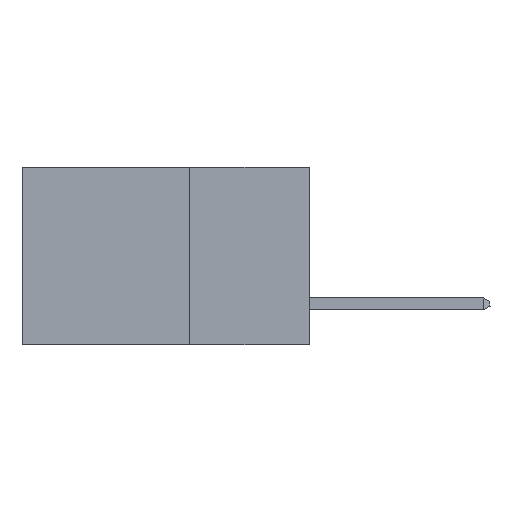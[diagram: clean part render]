
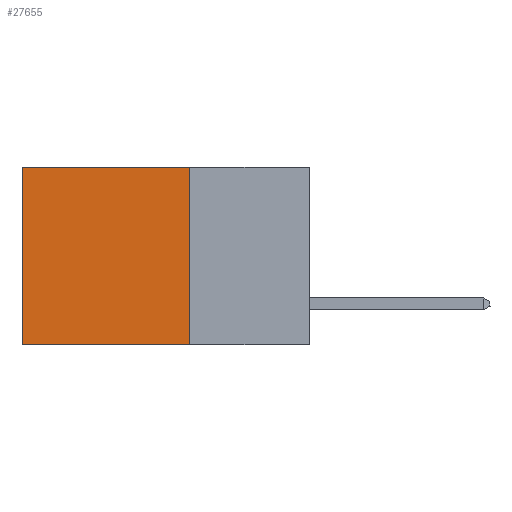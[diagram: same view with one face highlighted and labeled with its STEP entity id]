
A CAD part, left-side view. The second image highlights one B-rep face of the part: STEP entity #27655.
In plain terms, the highlighted planar face has unit normal (-1, 0, 0).
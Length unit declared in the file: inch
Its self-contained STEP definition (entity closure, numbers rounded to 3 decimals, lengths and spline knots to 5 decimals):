
#61 = LINE ( 'NONE', #29874, #7785 ) ;
#936 = EDGE_LOOP ( 'NONE', ( #32970, #7520, #23404, #4090 ) ) ;
#2208 = LINE ( 'NONE', #8037, #7498 ) ;
#3009 = VERTEX_POINT ( 'NONE', #13847 ) ;
#3869 = CARTESIAN_POINT ( 'NONE',  ( 0.2875, 0.25, -0.37 ) ) ;
#4090 = ORIENTED_EDGE ( 'NONE', *, *, #27673, .T. ) ;
#5864 = VECTOR ( 'NONE', #33023, 39.37008 ) ;
#5887 = AXIS2_PLACEMENT_3D ( 'NONE', #32640, #29722, #17159 ) ;
#6466 = VERTEX_POINT ( 'NONE', #9329 ) ;
#6578 = DIRECTION ( 'NONE',  ( 0., 1., 0. ) ) ;
#7107 = LINE ( 'NONE', #14974, #5864 ) ;
#7498 = VECTOR ( 'NONE', #31624, 39.37008 ) ;
#7520 = ORIENTED_EDGE ( 'NONE', *, *, #9804, .F. ) ;
#7785 = VECTOR ( 'NONE', #6578, 39.37008 ) ;
#8037 = CARTESIAN_POINT ( 'NONE',  ( 0.2875, 0.25, 0. ) ) ;
#8250 = LINE ( 'NONE', #16932, #19632 ) ;
#9329 = CARTESIAN_POINT ( 'NONE',  ( 0.2875, 0.6, 0. ) ) ;
#9804 = EDGE_CURVE ( 'NONE', #16215, #27872, #61, .T. ) ;
#13847 = CARTESIAN_POINT ( 'NONE',  ( 0.2875, 0.25, 0. ) ) ;
#14583 = PLANE ( 'NONE',  #5887 ) ;
#14974 = CARTESIAN_POINT ( 'NONE',  ( 0.2875, 0.6, 0. ) ) ;
#15435 = CARTESIAN_POINT ( 'NONE',  ( 0.2875, 0.6, -0.37 ) ) ;
#16208 = EDGE_CURVE ( 'NONE', #6466, #27872, #7107, .T. ) ;
#16215 = VERTEX_POINT ( 'NONE', #3869 ) ;
#16932 = CARTESIAN_POINT ( 'NONE',  ( 0.2875, 0.25, 0. ) ) ;
#17159 = DIRECTION ( 'NONE',  ( 0., 0., -1. ) ) ;
#17410 = EDGE_CURVE ( 'NONE', #3009, #16215, #2208, .T. ) ;
#19632 = VECTOR ( 'NONE', #27485, 39.37008 ) ;
#21205 = FACE_OUTER_BOUND ( 'NONE', #936, .T. ) ;
#23404 = ORIENTED_EDGE ( 'NONE', *, *, #17410, .F. ) ;
#27485 = DIRECTION ( 'NONE',  ( 0., 1., 0. ) ) ;
#27655 = ADVANCED_FACE ( 'NONE', ( #21205 ), #14583, .F. ) ;
#27673 = EDGE_CURVE ( 'NONE', #3009, #6466, #8250, .T. ) ;
#27872 = VERTEX_POINT ( 'NONE', #15435 ) ;
#29722 = DIRECTION ( 'NONE',  ( 1., 0., 0. ) ) ;
#29874 = CARTESIAN_POINT ( 'NONE',  ( 0.2875, 0.25, -0.37 ) ) ;
#31624 = DIRECTION ( 'NONE',  ( 0., 0., -1. ) ) ;
#32640 = CARTESIAN_POINT ( 'NONE',  ( 0.2875, 0.25, 0. ) ) ;
#32970 = ORIENTED_EDGE ( 'NONE', *, *, #16208, .T. ) ;
#33023 = DIRECTION ( 'NONE',  ( 0., 0., -1. ) ) ;
